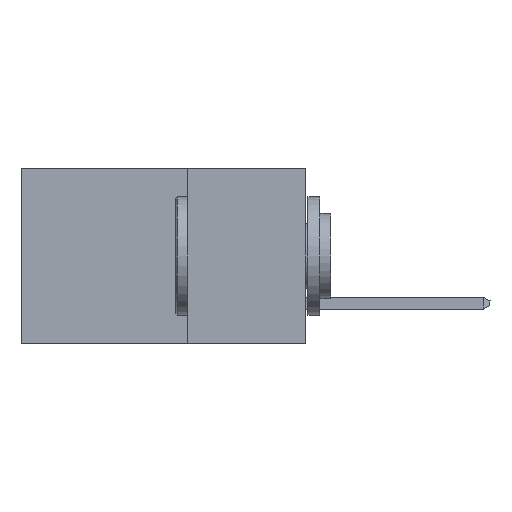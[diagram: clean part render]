
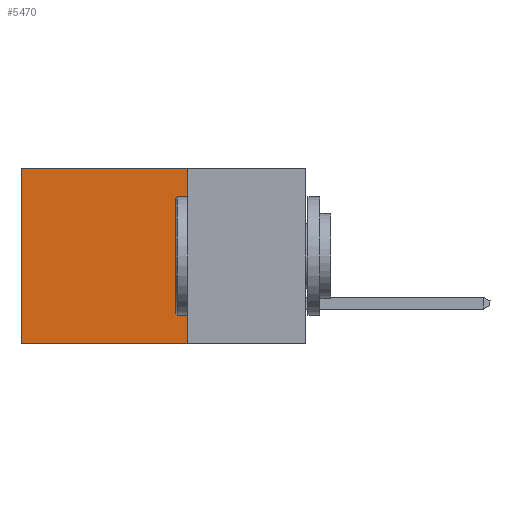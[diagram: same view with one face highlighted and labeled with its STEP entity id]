
A CAD part, left-side view. The second image highlights one B-rep face of the part: STEP entity #5470.
In plain terms, the highlighted planar face has unit normal (-1, 0, 0).
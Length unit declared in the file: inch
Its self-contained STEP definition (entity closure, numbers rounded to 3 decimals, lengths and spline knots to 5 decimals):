
#146 = CARTESIAN_POINT ( 'NONE',  ( 0.298, 0.6, 0. ) ) ;
#446 = DIRECTION ( 'NONE',  ( 0., 0., -1. ) ) ;
#1320 = EDGE_CURVE ( 'NONE', #11889, #12846, #11380, .T. ) ;
#2540 = PLANE ( 'NONE',  #6832 ) ;
#4063 = VECTOR ( 'NONE', #446, 39.37008 ) ;
#4685 = CARTESIAN_POINT ( 'NONE',  ( 0.298, 0.25, -0.37 ) ) ;
#5030 = DIRECTION ( 'NONE',  ( 0., 1., 0. ) ) ;
#5470 = ADVANCED_FACE ( 'NONE', ( #12014 ), #2540, .F. ) ;
#5520 = CARTESIAN_POINT ( 'NONE',  ( 0.298, 0.25, -0.37 ) ) ;
#5854 = VERTEX_POINT ( 'NONE', #14688 ) ;
#6445 = VECTOR ( 'NONE', #5030, 39.37008 ) ;
#6832 = AXIS2_PLACEMENT_3D ( 'NONE', #11462, #11519, #10326 ) ;
#7403 = LINE ( 'NONE', #14361, #4063 ) ;
#7989 = ORIENTED_EDGE ( 'NONE', *, *, #1320, .F. ) ;
#8263 = VERTEX_POINT ( 'NONE', #146 ) ;
#9376 = DIRECTION ( 'NONE',  ( 0., 1., 0. ) ) ;
#9654 = ORIENTED_EDGE ( 'NONE', *, *, #12752, .T. ) ;
#9662 = EDGE_CURVE ( 'NONE', #12846, #5854, #14334, .T. ) ;
#9821 = LINE ( 'NONE', #10055, #6445 ) ;
#10055 = CARTESIAN_POINT ( 'NONE',  ( 0.298, 0.25, 0. ) ) ;
#10146 = VECTOR ( 'NONE', #11657, 39.37008 ) ;
#10326 = DIRECTION ( 'NONE',  ( 0., 0., -1. ) ) ;
#11380 = LINE ( 'NONE', #13899, #10146 ) ;
#11462 = CARTESIAN_POINT ( 'NONE',  ( 0.298, 0.25, 0. ) ) ;
#11474 = EDGE_CURVE ( 'NONE', #11889, #8263, #9821, .T. ) ;
#11519 = DIRECTION ( 'NONE',  ( 1., 0., 0. ) ) ;
#11657 = DIRECTION ( 'NONE',  ( 0., 0., -1. ) ) ;
#11829 = EDGE_LOOP ( 'NONE', ( #9654, #15384, #7989, #12573 ) ) ;
#11889 = VERTEX_POINT ( 'NONE', #12826 ) ;
#12014 = FACE_OUTER_BOUND ( 'NONE', #11829, .T. ) ;
#12573 = ORIENTED_EDGE ( 'NONE', *, *, #11474, .T. ) ;
#12752 = EDGE_CURVE ( 'NONE', #8263, #5854, #7403, .T. ) ;
#12826 = CARTESIAN_POINT ( 'NONE',  ( 0.298, 0.25, 0. ) ) ;
#12846 = VERTEX_POINT ( 'NONE', #4685 ) ;
#13899 = CARTESIAN_POINT ( 'NONE',  ( 0.298, 0.25, 0. ) ) ;
#14334 = LINE ( 'NONE', #5520, #16324 ) ;
#14361 = CARTESIAN_POINT ( 'NONE',  ( 0.298, 0.6, 0. ) ) ;
#14688 = CARTESIAN_POINT ( 'NONE',  ( 0.298, 0.6, -0.37 ) ) ;
#15384 = ORIENTED_EDGE ( 'NONE', *, *, #9662, .F. ) ;
#16324 = VECTOR ( 'NONE', #9376, 39.37008 ) ;
